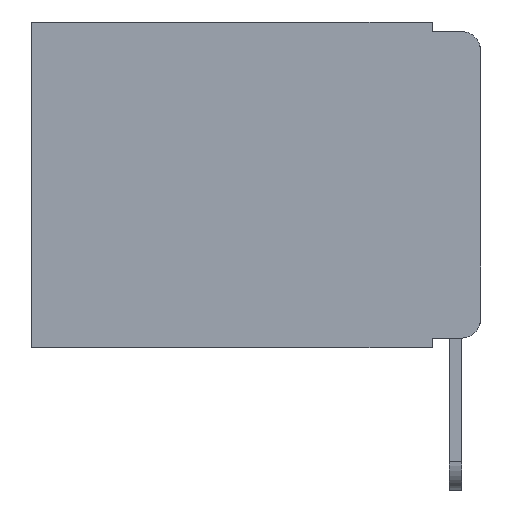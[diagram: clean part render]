
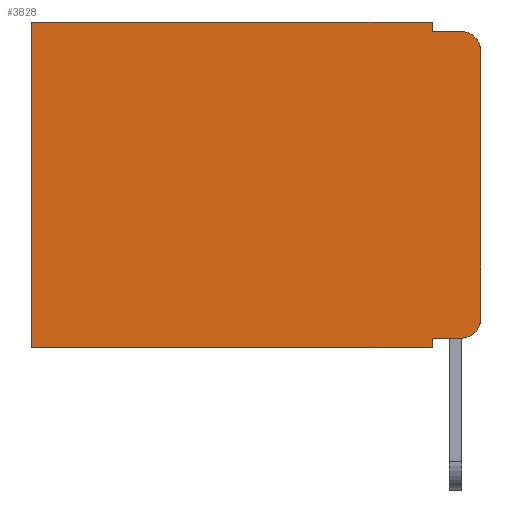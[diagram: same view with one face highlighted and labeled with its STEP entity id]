
A CAD part, left-side view. The second image highlights one B-rep face of the part: STEP entity #3828.
In plain terms, the highlighted planar face has unit normal (-1, 0, 0).
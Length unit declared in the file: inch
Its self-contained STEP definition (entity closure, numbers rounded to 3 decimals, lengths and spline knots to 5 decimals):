
#227 = ORIENTED_EDGE ( 'NONE', *, *, #9762, .T. ) ;
#827 = ORIENTED_EDGE ( 'NONE', *, *, #2813, .T. ) ;
#916 = VERTEX_POINT ( 'NONE', #4670 ) ;
#1199 = VECTOR ( 'NONE', #5725, 39.37008 ) ;
#1283 = CARTESIAN_POINT ( 'NONE',  ( 0.298, 0.02, -0.333 ) ) ;
#1299 = VERTEX_POINT ( 'NONE', #9679 ) ;
#1300 = CARTESIAN_POINT ( 'NONE',  ( 0.298, 0.051, -0.343 ) ) ;
#1368 = VERTEX_POINT ( 'NONE', #1300 ) ;
#1538 = VERTEX_POINT ( 'NONE', #8208 ) ;
#1952 = CARTESIAN_POINT ( 'NONE',  ( 0.298, 0., -0.313 ) ) ;
#2504 = ORIENTED_EDGE ( 'NONE', *, *, #8816, .F. ) ;
#2813 = EDGE_CURVE ( 'NONE', #1538, #916, #6553, .T. ) ;
#2936 = EDGE_LOOP ( 'NONE', ( #4824, #227, #9802, #2504, #5423, #827, #8500, #11219, #9079, #4993 ) ) ;
#2948 = VECTOR ( 'NONE', #6366, 39.37008 ) ;
#3187 = LINE ( 'NONE', #8039, #6074 ) ;
#3189 = DIRECTION ( 'NONE',  ( 0., 0., -1. ) ) ;
#3340 = CARTESIAN_POINT ( 'NONE',  ( 0.298, 0.051, 0. ) ) ;
#3359 = DIRECTION ( 'NONE',  ( 0., -1., 0. ) ) ;
#3387 = DIRECTION ( 'NONE',  ( 0., 0., -1. ) ) ;
#3569 = DIRECTION ( 'NONE',  ( -1., 0., 0. ) ) ;
#3799 = DIRECTION ( 'NONE',  ( 0., 0., -1. ) ) ;
#3816 = LINE ( 'NONE', #11284, #1199 ) ;
#3828 = ADVANCED_FACE ( 'NONE', ( #9529 ), #12062, .F. ) ;
#4328 = EDGE_CURVE ( 'NONE', #1299, #7816, #9958, .T. ) ;
#4414 = DIRECTION ( 'NONE',  ( -1., 0., 0. ) ) ;
#4670 = CARTESIAN_POINT ( 'NONE',  ( 0.298, 0.473, -0.343 ) ) ;
#4796 = CARTESIAN_POINT ( 'NONE',  ( 0.298, 0.473, 0. ) ) ;
#4824 = ORIENTED_EDGE ( 'NONE', *, *, #7784, .F. ) ;
#4993 = ORIENTED_EDGE ( 'NONE', *, *, #5839, .T. ) ;
#5361 = AXIS2_PLACEMENT_3D ( 'NONE', #9652, #10088, #11079 ) ;
#5423 = ORIENTED_EDGE ( 'NONE', *, *, #10184, .T. ) ;
#5540 = CARTESIAN_POINT ( 'NONE',  ( 0.298, 0.02, -0.313 ) ) ;
#5616 = LINE ( 'NONE', #3340, #7513 ) ;
#5725 = DIRECTION ( 'NONE',  ( 0., 0., -1. ) ) ;
#5814 = VERTEX_POINT ( 'NONE', #9410 ) ;
#5839 = EDGE_CURVE ( 'NONE', #7816, #12008, #9499, .T. ) ;
#5967 = VERTEX_POINT ( 'NONE', #7903 ) ;
#6074 = VECTOR ( 'NONE', #8988, 39.37008 ) ;
#6183 = CARTESIAN_POINT ( 'NONE',  ( 0.298, 0.051, -0.01 ) ) ;
#6252 = CARTESIAN_POINT ( 'NONE',  ( 0.298, 0.051, -0.333 ) ) ;
#6366 = DIRECTION ( 'NONE',  ( 0., -1., 0. ) ) ;
#6553 = LINE ( 'NONE', #4796, #10664 ) ;
#6951 = VECTOR ( 'NONE', #3189, 39.37008 ) ;
#7292 = AXIS2_PLACEMENT_3D ( 'NONE', #5540, #4414, #3387 ) ;
#7297 = EDGE_CURVE ( 'NONE', #1368, #916, #11309, .T. ) ;
#7347 = CARTESIAN_POINT ( 'NONE',  ( 0.298, 0., -0.343 ) ) ;
#7377 = LINE ( 'NONE', #9052, #11959 ) ;
#7513 = VECTOR ( 'NONE', #8094, 39.37008 ) ;
#7784 = EDGE_CURVE ( 'NONE', #5967, #12008, #9445, .T. ) ;
#7816 = VERTEX_POINT ( 'NONE', #1283 ) ;
#7903 = CARTESIAN_POINT ( 'NONE',  ( 0.298, 0., -0.03 ) ) ;
#8039 = CARTESIAN_POINT ( 'NONE',  ( 0.298, 0., 0. ) ) ;
#8094 = DIRECTION ( 'NONE',  ( 0., 0., -1. ) ) ;
#8208 = CARTESIAN_POINT ( 'NONE',  ( 0.298, 0.473, 0. ) ) ;
#8435 = VERTEX_POINT ( 'NONE', #6183 ) ;
#8500 = ORIENTED_EDGE ( 'NONE', *, *, #7297, .F. ) ;
#8505 = EDGE_CURVE ( 'NONE', #8435, #10875, #7377, .T. ) ;
#8816 = EDGE_CURVE ( 'NONE', #5814, #8435, #3816, .T. ) ;
#8871 = VECTOR ( 'NONE', #11043, 39.37008 ) ;
#8889 = CARTESIAN_POINT ( 'NONE',  ( 0.298, 0., 0. ) ) ;
#8988 = DIRECTION ( 'NONE',  ( 0., 1., 0. ) ) ;
#9014 = CARTESIAN_POINT ( 'NONE',  ( 0.298, 0.02, -0.01 ) ) ;
#9052 = CARTESIAN_POINT ( 'NONE',  ( 0.298, 0.051, -0.01 ) ) ;
#9079 = ORIENTED_EDGE ( 'NONE', *, *, #4328, .T. ) ;
#9207 = EDGE_CURVE ( 'NONE', #1299, #1368, #5616, .T. ) ;
#9236 = CARTESIAN_POINT ( 'NONE',  ( 0.298, 0.02, -0.03 ) ) ;
#9410 = CARTESIAN_POINT ( 'NONE',  ( 0.298, 0.051, 0. ) ) ;
#9445 = LINE ( 'NONE', #8889, #6951 ) ;
#9499 = CIRCLE ( 'NONE', #7292, 0.02 ) ;
#9529 = FACE_OUTER_BOUND ( 'NONE', #2936, .T. ) ;
#9652 = CARTESIAN_POINT ( 'NONE',  ( 0.298, 0., 0. ) ) ;
#9679 = CARTESIAN_POINT ( 'NONE',  ( 0.298, 0.051, -0.333 ) ) ;
#9762 = EDGE_CURVE ( 'NONE', #5967, #10875, #11800, .T. ) ;
#9802 = ORIENTED_EDGE ( 'NONE', *, *, #8505, .F. ) ;
#9958 = LINE ( 'NONE', #6252, #2948 ) ;
#10088 = DIRECTION ( 'NONE',  ( 1., 0., 0. ) ) ;
#10184 = EDGE_CURVE ( 'NONE', #5814, #1538, #3187, .T. ) ;
#10196 = DIRECTION ( 'NONE',  ( 0., 0., -1. ) ) ;
#10405 = AXIS2_PLACEMENT_3D ( 'NONE', #9236, #3569, #10196 ) ;
#10664 = VECTOR ( 'NONE', #3799, 39.37008 ) ;
#10875 = VERTEX_POINT ( 'NONE', #9014 ) ;
#11043 = DIRECTION ( 'NONE',  ( 0., 1., 0. ) ) ;
#11079 = DIRECTION ( 'NONE',  ( 0., 0., -1. ) ) ;
#11219 = ORIENTED_EDGE ( 'NONE', *, *, #9207, .F. ) ;
#11284 = CARTESIAN_POINT ( 'NONE',  ( 0.298, 0.051, 0. ) ) ;
#11309 = LINE ( 'NONE', #7347, #8871 ) ;
#11800 = CIRCLE ( 'NONE', #10405, 0.02 ) ;
#11959 = VECTOR ( 'NONE', #3359, 39.37008 ) ;
#12008 = VERTEX_POINT ( 'NONE', #1952 ) ;
#12062 = PLANE ( 'NONE',  #5361 ) ;
